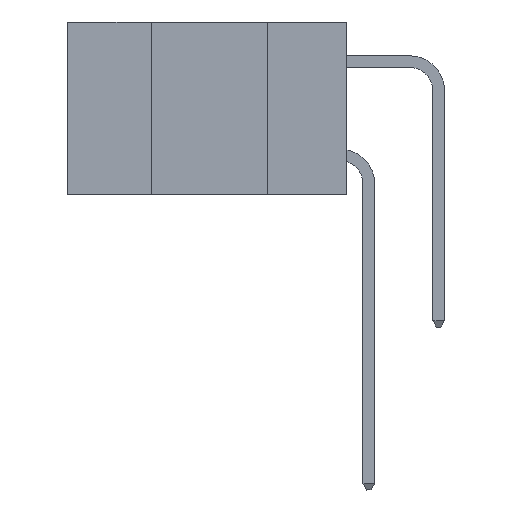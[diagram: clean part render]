
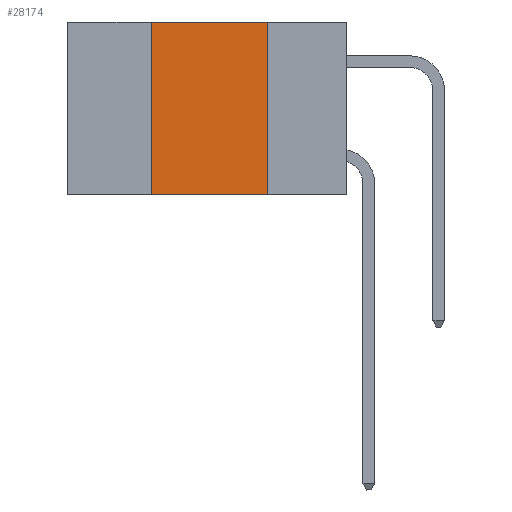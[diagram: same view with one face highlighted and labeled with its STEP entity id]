
A CAD part, left-side view. The second image highlights one B-rep face of the part: STEP entity #28174.
In plain terms, the highlighted planar face has unit normal (-1, 0, 0).
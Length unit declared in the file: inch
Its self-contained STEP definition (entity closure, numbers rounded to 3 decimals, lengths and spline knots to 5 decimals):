
#23 = DIRECTION ( 'NONE',  ( 0., 0., 1. ) ) ;
#354 = EDGE_CURVE ( 'NONE', #24823, #10755, #19812, .T. ) ;
#867 = LINE ( 'NONE', #15628, #13243 ) ;
#2133 = DIRECTION ( 'NONE',  ( 1., 0., 0. ) ) ;
#2312 = FACE_OUTER_BOUND ( 'NONE', #6040, .T. ) ;
#4025 = DIRECTION ( 'NONE',  ( 0., -1., 0. ) ) ;
#4915 = DIRECTION ( 'NONE',  ( 0., 0., -1. ) ) ;
#5095 = VECTOR ( 'NONE', #4025, 39.37008 ) ;
#5818 = PLANE ( 'NONE',  #11806 ) ;
#6040 = EDGE_LOOP ( 'NONE', ( #17374, #12835, #11373, #8983 ) ) ;
#6301 = VERTEX_POINT ( 'NONE', #28013 ) ;
#7493 = VECTOR ( 'NONE', #29541, 39.37008 ) ;
#8983 = ORIENTED_EDGE ( 'NONE', *, *, #354, .T. ) ;
#10258 = EDGE_CURVE ( 'NONE', #6301, #10755, #27288, .T. ) ;
#10707 = LINE ( 'NONE', #18975, #19994 ) ;
#10755 = VERTEX_POINT ( 'NONE', #16718 ) ;
#11373 = ORIENTED_EDGE ( 'NONE', *, *, #25434, .F. ) ;
#11660 = CARTESIAN_POINT ( 'NONE',  ( 0., 0.6, 0. ) ) ;
#11806 = AXIS2_PLACEMENT_3D ( 'NONE', #11660, #2133, #4915 ) ;
#12835 = ORIENTED_EDGE ( 'NONE', *, *, #16263, .F. ) ;
#13243 = VECTOR ( 'NONE', #26080, 39.37008 ) ;
#14369 = CARTESIAN_POINT ( 'NONE',  ( 0., 0.42, 0. ) ) ;
#15628 = CARTESIAN_POINT ( 'NONE',  ( 0., 0.6, 0. ) ) ;
#16263 = EDGE_CURVE ( 'NONE', #22733, #6301, #867, .T. ) ;
#16718 = CARTESIAN_POINT ( 'NONE',  ( 0., 0.17, -0.37 ) ) ;
#17374 = ORIENTED_EDGE ( 'NONE', *, *, #10258, .F. ) ;
#18975 = CARTESIAN_POINT ( 'NONE',  ( 0., 0.42, 0. ) ) ;
#19234 = CARTESIAN_POINT ( 'NONE',  ( 0., 0.42, -0.37 ) ) ;
#19284 = CARTESIAN_POINT ( 'NONE',  ( 0., 0.6, -0.37 ) ) ;
#19812 = LINE ( 'NONE', #19284, #5095 ) ;
#19994 = VECTOR ( 'NONE', #23, 39.37008 ) ;
#22733 = VERTEX_POINT ( 'NONE', #14369 ) ;
#24595 = CARTESIAN_POINT ( 'NONE',  ( 0., 0.17, 0. ) ) ;
#24823 = VERTEX_POINT ( 'NONE', #19234 ) ;
#25434 = EDGE_CURVE ( 'NONE', #24823, #22733, #10707, .T. ) ;
#26080 = DIRECTION ( 'NONE',  ( 0., -1., 0. ) ) ;
#27288 = LINE ( 'NONE', #24595, #7493 ) ;
#28013 = CARTESIAN_POINT ( 'NONE',  ( 0., 0.17, 0. ) ) ;
#28174 = ADVANCED_FACE ( 'NONE', ( #2312 ), #5818, .F. ) ;
#29541 = DIRECTION ( 'NONE',  ( 0., 0., -1. ) ) ;
